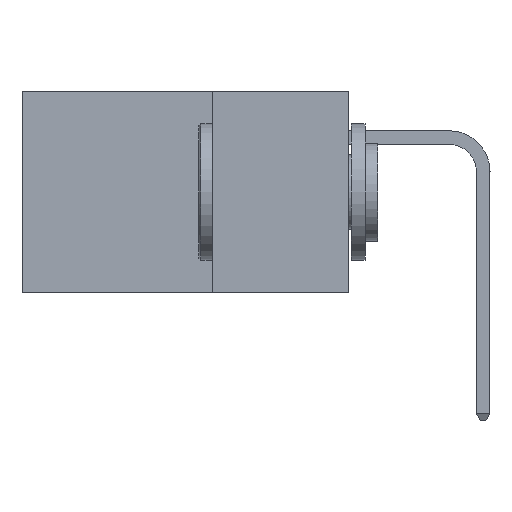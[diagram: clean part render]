
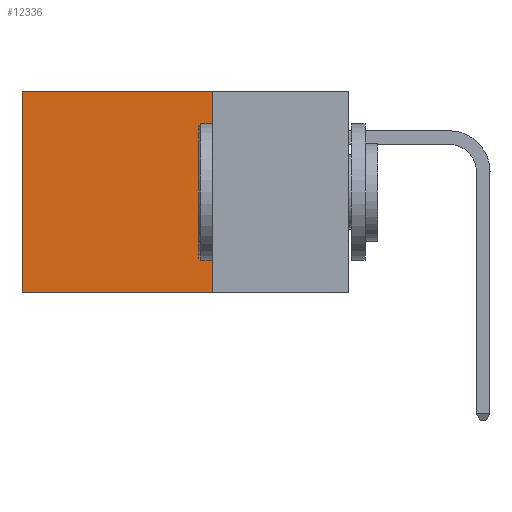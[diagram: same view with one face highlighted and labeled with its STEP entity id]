
A CAD part, left-side view. The second image highlights one B-rep face of the part: STEP entity #12336.
In plain terms, the highlighted planar face has unit normal (-1, 0, 0).
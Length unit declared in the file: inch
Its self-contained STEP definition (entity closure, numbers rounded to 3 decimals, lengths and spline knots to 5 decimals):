
#487 = VERTEX_POINT ( 'NONE', #15728 ) ;
#544 = VECTOR ( 'NONE', #4246, 39.37008 ) ;
#1465 = VECTOR ( 'NONE', #5887, 39.37008 ) ;
#1985 = DIRECTION ( 'NONE',  ( 0., 0., -1. ) ) ;
#3237 = ORIENTED_EDGE ( 'NONE', *, *, #31743, .F. ) ;
#4246 = DIRECTION ( 'NONE',  ( 0., 0., -1. ) ) ;
#4361 = ORIENTED_EDGE ( 'NONE', *, *, #6094, .T. ) ;
#5887 = DIRECTION ( 'NONE',  ( 0., 1., 0. ) ) ;
#6094 = EDGE_CURVE ( 'NONE', #10889, #487, #39311, .T. ) ;
#7131 = EDGE_LOOP ( 'NONE', ( #4361, #3237, #10394, #27162 ) ) ;
#10282 = CARTESIAN_POINT ( 'NONE',  ( 0.2875, 0.25, -0.37 ) ) ;
#10394 = ORIENTED_EDGE ( 'NONE', *, *, #18077, .F. ) ;
#10889 = VERTEX_POINT ( 'NONE', #14891 ) ;
#11883 = CARTESIAN_POINT ( 'NONE',  ( 0.2875, 0.25, 0. ) ) ;
#12336 = ADVANCED_FACE ( 'NONE', ( #21276 ), #31978, .F. ) ;
#13019 = CARTESIAN_POINT ( 'NONE',  ( 0.2875, 0.25, -0.37 ) ) ;
#14891 = CARTESIAN_POINT ( 'NONE',  ( 0.2875, 0.6, 0. ) ) ;
#15507 = CARTESIAN_POINT ( 'NONE',  ( 0.2875, 0.25, 0. ) ) ;
#15728 = CARTESIAN_POINT ( 'NONE',  ( 0.2875, 0.6, -0.37 ) ) ;
#18077 = EDGE_CURVE ( 'NONE', #41724, #19110, #36892, .T. ) ;
#18849 = DIRECTION ( 'NONE',  ( 0., 0., -1. ) ) ;
#19110 = VERTEX_POINT ( 'NONE', #13019 ) ;
#20864 = CARTESIAN_POINT ( 'NONE',  ( 0.2875, 0.25, 0. ) ) ;
#21276 = FACE_OUTER_BOUND ( 'NONE', #7131, .T. ) ;
#27162 = ORIENTED_EDGE ( 'NONE', *, *, #40554, .T. ) ;
#29077 = CARTESIAN_POINT ( 'NONE',  ( 0.2875, 0.25, 0. ) ) ;
#29319 = LINE ( 'NONE', #10282, #39099 ) ;
#29550 = VECTOR ( 'NONE', #1985, 39.37008 ) ;
#31743 = EDGE_CURVE ( 'NONE', #19110, #487, #29319, .T. ) ;
#31753 = CARTESIAN_POINT ( 'NONE',  ( 0.2875, 0.6, 0. ) ) ;
#31978 = PLANE ( 'NONE',  #40886 ) ;
#33458 = DIRECTION ( 'NONE',  ( 0., 1., 0. ) ) ;
#35711 = LINE ( 'NONE', #29077, #1465 ) ;
#36892 = LINE ( 'NONE', #20864, #544 ) ;
#38600 = DIRECTION ( 'NONE',  ( 1., 0., 0. ) ) ;
#39099 = VECTOR ( 'NONE', #33458, 39.37008 ) ;
#39311 = LINE ( 'NONE', #31753, #29550 ) ;
#40554 = EDGE_CURVE ( 'NONE', #41724, #10889, #35711, .T. ) ;
#40886 = AXIS2_PLACEMENT_3D ( 'NONE', #15507, #38600, #18849 ) ;
#41724 = VERTEX_POINT ( 'NONE', #11883 ) ;
